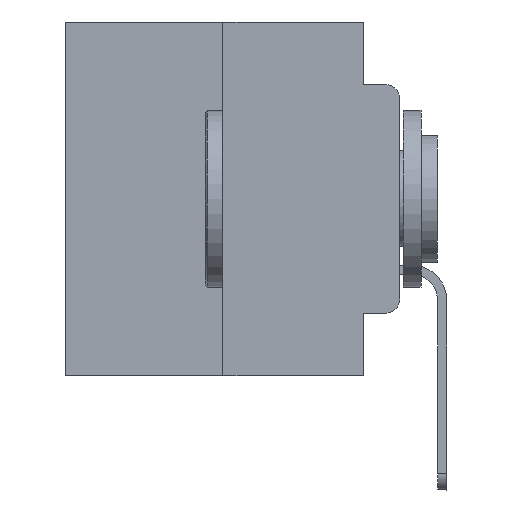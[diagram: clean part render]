
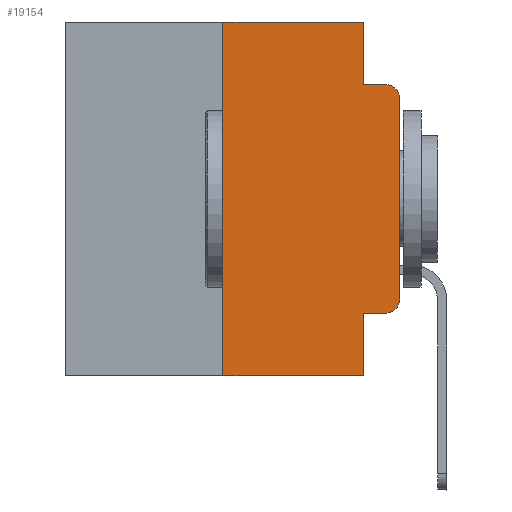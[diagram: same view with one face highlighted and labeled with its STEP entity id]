
A CAD part, left-side view. The second image highlights one B-rep face of the part: STEP entity #19154.
In plain terms, the highlighted planar face has unit normal (-1, 0, 0).
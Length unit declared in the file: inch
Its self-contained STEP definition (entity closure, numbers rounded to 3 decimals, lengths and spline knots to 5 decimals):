
#391 = EDGE_CURVE ( 'NONE', #14520, #12529, #16788, .T. ) ;
#760 = LINE ( 'NONE', #19140, #10137 ) ;
#908 = CARTESIAN_POINT ( 'NONE',  ( 0., 0.051, -0.5 ) ) ;
#1400 = LINE ( 'NONE', #19769, #21474 ) ;
#1421 = LINE ( 'NONE', #22746, #22915 ) ;
#1841 = CARTESIAN_POINT ( 'NONE',  ( 0., 0.051, 0. ) ) ;
#2725 = VERTEX_POINT ( 'NONE', #1841 ) ;
#3297 = EDGE_CURVE ( 'NONE', #2725, #10949, #8743, .T. ) ;
#3348 = DIRECTION ( 'NONE',  ( 0., -1., 0. ) ) ;
#4070 = VECTOR ( 'NONE', #23158, 39.37008 ) ;
#4285 = CARTESIAN_POINT ( 'NONE',  ( 0., 0., 0. ) ) ;
#4956 = VECTOR ( 'NONE', #23466, 39.37008 ) ;
#5028 = CIRCLE ( 'NONE', #12856, 0.02 ) ;
#5123 = DIRECTION ( 'NONE',  ( 0., 0., -1. ) ) ;
#6553 = VERTEX_POINT ( 'NONE', #26115 ) ;
#6951 = VERTEX_POINT ( 'NONE', #9829 ) ;
#6960 = CARTESIAN_POINT ( 'NONE',  ( 0., 0.473, 0. ) ) ;
#7110 = CARTESIAN_POINT ( 'NONE',  ( 0., 0.051, -0.0885 ) ) ;
#7297 = ORIENTED_EDGE ( 'NONE', *, *, #9968, .T. ) ;
#8028 = CARTESIAN_POINT ( 'NONE',  ( 0., 0.473, 0. ) ) ;
#8743 = LINE ( 'NONE', #25328, #4070 ) ;
#8978 = ORIENTED_EDGE ( 'NONE', *, *, #24228, .F. ) ;
#9435 = EDGE_CURVE ( 'NONE', #15833, #13947, #760, .T. ) ;
#9829 = CARTESIAN_POINT ( 'NONE',  ( 0., 0.25, 0. ) ) ;
#9875 = AXIS2_PLACEMENT_3D ( 'NONE', #6960, #10776, #20609 ) ;
#9890 = ORIENTED_EDGE ( 'NONE', *, *, #18300, .F. ) ;
#9968 = EDGE_CURVE ( 'NONE', #13527, #13947, #1400, .T. ) ;
#10137 = VECTOR ( 'NONE', #5123, 39.37008 ) ;
#10591 = CARTESIAN_POINT ( 'NONE',  ( 0., 0.02, -0.1085 ) ) ;
#10696 = AXIS2_PLACEMENT_3D ( 'NONE', #18387, #22736, #18528 ) ;
#10776 = DIRECTION ( 'NONE',  ( 1., 0., 0. ) ) ;
#10925 = CARTESIAN_POINT ( 'NONE',  ( 0., 0.25, -0.5 ) ) ;
#10949 = VERTEX_POINT ( 'NONE', #7110 ) ;
#11100 = CARTESIAN_POINT ( 'NONE',  ( 0., 0.02, -0.0885 ) ) ;
#11576 = VECTOR ( 'NONE', #12251, 39.37008 ) ;
#12186 = LINE ( 'NONE', #4285, #20230 ) ;
#12251 = DIRECTION ( 'NONE',  ( 0., -1., 0. ) ) ;
#12377 = LINE ( 'NONE', #8028, #11576 ) ;
#12529 = VERTEX_POINT ( 'NONE', #17821 ) ;
#12856 = AXIS2_PLACEMENT_3D ( 'NONE', #10591, #25029, #15078 ) ;
#13204 = PLANE ( 'NONE',  #9875 ) ;
#13236 = LINE ( 'NONE', #17194, #4956 ) ;
#13527 = VERTEX_POINT ( 'NONE', #10925 ) ;
#13947 = VERTEX_POINT ( 'NONE', #908 ) ;
#14369 = ORIENTED_EDGE ( 'NONE', *, *, #18969, .F. ) ;
#14520 = VERTEX_POINT ( 'NONE', #22245 ) ;
#14706 = ORIENTED_EDGE ( 'NONE', *, *, #391, .T. ) ;
#15078 = DIRECTION ( 'NONE',  ( 0., 0., -1. ) ) ;
#15181 = CARTESIAN_POINT ( 'NONE',  ( 0., 0.051, -0.4115 ) ) ;
#15833 = VERTEX_POINT ( 'NONE', #15181 ) ;
#15878 = VERTEX_POINT ( 'NONE', #11100 ) ;
#16788 = CIRCLE ( 'NONE', #10696, 0.02 ) ;
#17194 = CARTESIAN_POINT ( 'NONE',  ( 0., 0.051, -0.0885 ) ) ;
#17466 = EDGE_CURVE ( 'NONE', #12529, #6553, #12186, .T. ) ;
#17821 = CARTESIAN_POINT ( 'NONE',  ( 0., 0., -0.3915 ) ) ;
#18185 = DIRECTION ( 'NONE',  ( 0., 0., 1. ) ) ;
#18300 = EDGE_CURVE ( 'NONE', #6951, #2725, #12377, .T. ) ;
#18313 = LINE ( 'NONE', #18438, #19733 ) ;
#18387 = CARTESIAN_POINT ( 'NONE',  ( 0., 0.02, -0.3915 ) ) ;
#18438 = CARTESIAN_POINT ( 'NONE',  ( 0., 0.051, -0.4115 ) ) ;
#18528 = DIRECTION ( 'NONE',  ( 0., 0., -1. ) ) ;
#18793 = DIRECTION ( 'NONE',  ( 0., 0., 1. ) ) ;
#18969 = EDGE_CURVE ( 'NONE', #13527, #6951, #1421, .T. ) ;
#19140 = CARTESIAN_POINT ( 'NONE',  ( 0., 0.051, 0. ) ) ;
#19154 = ADVANCED_FACE ( 'NONE', ( #25597 ), #13204, .F. ) ;
#19556 = EDGE_CURVE ( 'NONE', #6553, #15878, #5028, .T. ) ;
#19733 = VECTOR ( 'NONE', #3348, 39.37008 ) ;
#19769 = CARTESIAN_POINT ( 'NONE',  ( 0., 0.473, -0.5 ) ) ;
#20050 = DIRECTION ( 'NONE',  ( 0., -1., 0. ) ) ;
#20098 = ORIENTED_EDGE ( 'NONE', *, *, #3297, .F. ) ;
#20230 = VECTOR ( 'NONE', #18185, 39.37008 ) ;
#20609 = DIRECTION ( 'NONE',  ( 0., 0., -1. ) ) ;
#20656 = ORIENTED_EDGE ( 'NONE', *, *, #23055, .T. ) ;
#20704 = ORIENTED_EDGE ( 'NONE', *, *, #17466, .T. ) ;
#21474 = VECTOR ( 'NONE', #20050, 39.37008 ) ;
#22245 = CARTESIAN_POINT ( 'NONE',  ( 0., 0.02, -0.4115 ) ) ;
#22736 = DIRECTION ( 'NONE',  ( -1., 0., 0. ) ) ;
#22746 = CARTESIAN_POINT ( 'NONE',  ( 0., 0.25, 0. ) ) ;
#22915 = VECTOR ( 'NONE', #18793, 39.37008 ) ;
#23055 = EDGE_CURVE ( 'NONE', #15833, #14520, #18313, .T. ) ;
#23158 = DIRECTION ( 'NONE',  ( 0., 0., -1. ) ) ;
#23464 = ORIENTED_EDGE ( 'NONE', *, *, #9435, .F. ) ;
#23466 = DIRECTION ( 'NONE',  ( 0., -1., 0. ) ) ;
#24228 = EDGE_CURVE ( 'NONE', #10949, #15878, #13236, .T. ) ;
#25029 = DIRECTION ( 'NONE',  ( -1., 0., 0. ) ) ;
#25049 = EDGE_LOOP ( 'NONE', ( #20704, #25266, #8978, #20098, #9890, #14369, #7297, #23464, #20656, #14706 ) ) ;
#25266 = ORIENTED_EDGE ( 'NONE', *, *, #19556, .T. ) ;
#25328 = CARTESIAN_POINT ( 'NONE',  ( 0., 0.051, 0. ) ) ;
#25597 = FACE_OUTER_BOUND ( 'NONE', #25049, .T. ) ;
#26115 = CARTESIAN_POINT ( 'NONE',  ( 0., 0., -0.1085 ) ) ;
